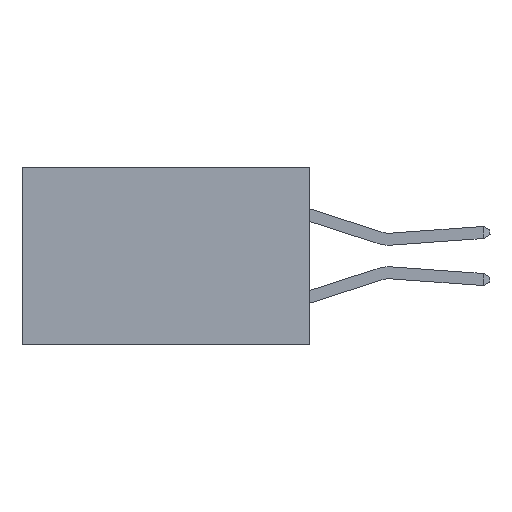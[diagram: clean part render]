
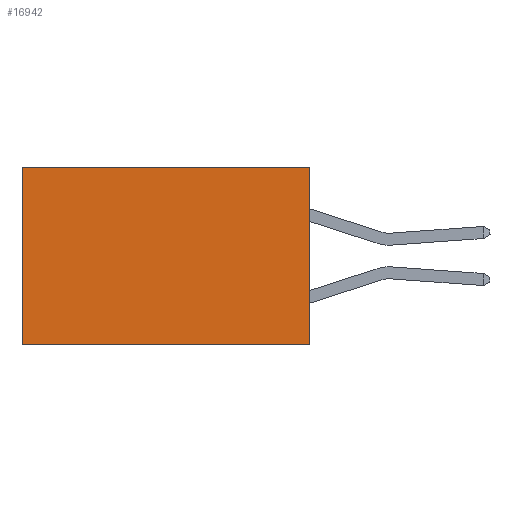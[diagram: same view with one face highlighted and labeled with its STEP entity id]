
A CAD part, left-side view. The second image highlights one B-rep face of the part: STEP entity #16942.
In plain terms, the highlighted planar face has unit normal (-1, 0, 0).
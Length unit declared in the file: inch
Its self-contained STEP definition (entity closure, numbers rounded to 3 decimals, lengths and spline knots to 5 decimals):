
#33 = ORIENTED_EDGE ( 'NONE', *, *, #9100, .T. ) ;
#528 = DIRECTION ( 'NONE',  ( 0., 1., 0. ) ) ;
#1392 = VERTEX_POINT ( 'NONE', #17588 ) ;
#1458 = DIRECTION ( 'NONE',  ( 0., 0., -1. ) ) ;
#2155 = VERTEX_POINT ( 'NONE', #18897 ) ;
#2556 = ORIENTED_EDGE ( 'NONE', *, *, #8073, .F. ) ;
#4682 = CARTESIAN_POINT ( 'NONE',  ( 0.298, 0., 0. ) ) ;
#5859 = DIRECTION ( 'NONE',  ( 0., 0., -1. ) ) ;
#6153 = CARTESIAN_POINT ( 'NONE',  ( 0.298, 0.6, 0. ) ) ;
#8073 = EDGE_CURVE ( 'NONE', #21241, #2155, #22131, .T. ) ;
#9100 = EDGE_CURVE ( 'NONE', #1392, #2155, #19780, .T. ) ;
#9531 = ORIENTED_EDGE ( 'NONE', *, *, #19256, .T. ) ;
#9683 = CARTESIAN_POINT ( 'NONE',  ( 0.298, 0., 0. ) ) ;
#11434 = CARTESIAN_POINT ( 'NONE',  ( 0.298, 0., -0.37 ) ) ;
#11584 = EDGE_CURVE ( 'NONE', #25026, #21241, #18417, .T. ) ;
#12529 = AXIS2_PLACEMENT_3D ( 'NONE', #9683, #13803, #1458 ) ;
#12793 = VECTOR ( 'NONE', #528, 39.37008 ) ;
#12948 = VECTOR ( 'NONE', #5859, 39.37008 ) ;
#13287 = EDGE_LOOP ( 'NONE', ( #33, #2556, #16146, #9531 ) ) ;
#13690 = VECTOR ( 'NONE', #18455, 39.37008 ) ;
#13803 = DIRECTION ( 'NONE',  ( 1., 0., 0. ) ) ;
#16146 = ORIENTED_EDGE ( 'NONE', *, *, #11584, .F. ) ;
#16269 = DIRECTION ( 'NONE',  ( 0., 1., 0. ) ) ;
#16942 = ADVANCED_FACE ( 'NONE', ( #25999 ), #17846, .F. ) ;
#17588 = CARTESIAN_POINT ( 'NONE',  ( 0.298, 0.6, 0. ) ) ;
#17846 = PLANE ( 'NONE',  #12529 ) ;
#18417 = LINE ( 'NONE', #22113, #12948 ) ;
#18455 = DIRECTION ( 'NONE',  ( 0., 0., -1. ) ) ;
#18897 = CARTESIAN_POINT ( 'NONE',  ( 0.298, 0.6, -0.37 ) ) ;
#19256 = EDGE_CURVE ( 'NONE', #25026, #1392, #23080, .T. ) ;
#19780 = LINE ( 'NONE', #6153, #13690 ) ;
#20425 = CARTESIAN_POINT ( 'NONE',  ( 0.298, 0., -0.37 ) ) ;
#21241 = VERTEX_POINT ( 'NONE', #11434 ) ;
#21681 = CARTESIAN_POINT ( 'NONE',  ( 0.298, 0., 0. ) ) ;
#22113 = CARTESIAN_POINT ( 'NONE',  ( 0.298, 0., 0. ) ) ;
#22131 = LINE ( 'NONE', #20425, #26248 ) ;
#23080 = LINE ( 'NONE', #4682, #12793 ) ;
#25026 = VERTEX_POINT ( 'NONE', #21681 ) ;
#25999 = FACE_OUTER_BOUND ( 'NONE', #13287, .T. ) ;
#26248 = VECTOR ( 'NONE', #16269, 39.37008 ) ;
